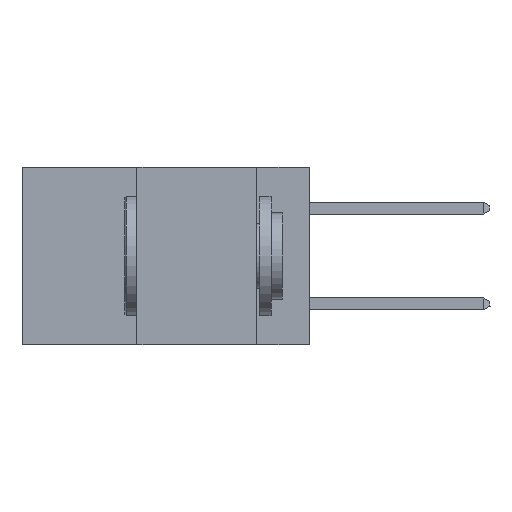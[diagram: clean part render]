
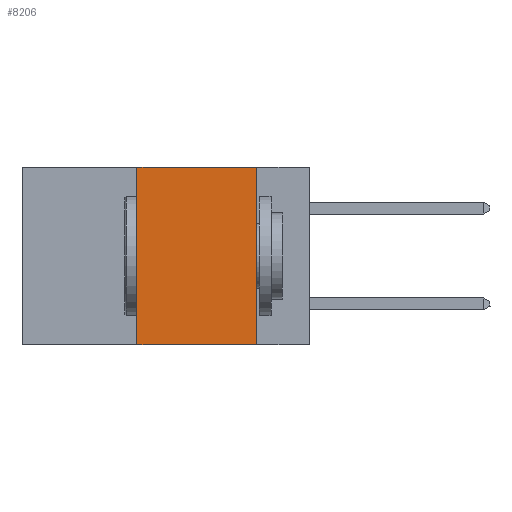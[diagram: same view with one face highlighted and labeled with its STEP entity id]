
A CAD part, left-side view. The second image highlights one B-rep face of the part: STEP entity #8206.
In plain terms, the highlighted planar face has unit normal (-1, 0, 0).
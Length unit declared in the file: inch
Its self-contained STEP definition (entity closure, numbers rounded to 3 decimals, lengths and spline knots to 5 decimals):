
#815 = VECTOR ( 'NONE', #8170, 39.37008 ) ;
#894 = VECTOR ( 'NONE', #13691, 39.37008 ) ;
#2569 = VECTOR ( 'NONE', #21278, 39.37008 ) ;
#2693 = CARTESIAN_POINT ( 'NONE',  ( 0., 0.6, -0.37 ) ) ;
#2923 = EDGE_CURVE ( 'NONE', #23876, #13328, #21551, .T. ) ;
#3193 = LINE ( 'NONE', #19257, #2569 ) ;
#3829 = CARTESIAN_POINT ( 'NONE',  ( 0., 0.6, 0. ) ) ;
#5627 = DIRECTION ( 'NONE',  ( 1., 0., 0. ) ) ;
#5824 = EDGE_CURVE ( 'NONE', #13328, #7468, #11287, .T. ) ;
#6142 = EDGE_CURVE ( 'NONE', #23876, #15051, #16605, .T. ) ;
#7190 = CARTESIAN_POINT ( 'NONE',  ( 0., 0.11, 0. ) ) ;
#7249 = ORIENTED_EDGE ( 'NONE', *, *, #15564, .F. ) ;
#7383 = CARTESIAN_POINT ( 'NONE',  ( 0., 0.36, 0. ) ) ;
#7468 = VERTEX_POINT ( 'NONE', #7190 ) ;
#8170 = DIRECTION ( 'NONE',  ( 0., 0., 1. ) ) ;
#8206 = ADVANCED_FACE ( 'NONE', ( #18088 ), #23444, .F. ) ;
#9370 = CARTESIAN_POINT ( 'NONE',  ( 0., 0.6, 0. ) ) ;
#10376 = CARTESIAN_POINT ( 'NONE',  ( 0., 0.36, 0. ) ) ;
#10899 = ORIENTED_EDGE ( 'NONE', *, *, #5824, .F. ) ;
#11287 = LINE ( 'NONE', #3829, #894 ) ;
#12989 = AXIS2_PLACEMENT_3D ( 'NONE', #9370, #5627, #19761 ) ;
#13328 = VERTEX_POINT ( 'NONE', #7383 ) ;
#13691 = DIRECTION ( 'NONE',  ( 0., -1., 0. ) ) ;
#14237 = CARTESIAN_POINT ( 'NONE',  ( 0., 0.36, -0.37 ) ) ;
#15051 = VERTEX_POINT ( 'NONE', #25964 ) ;
#15564 = EDGE_CURVE ( 'NONE', #7468, #15051, #3193, .T. ) ;
#16605 = LINE ( 'NONE', #2693, #18790 ) ;
#16943 = ORIENTED_EDGE ( 'NONE', *, *, #2923, .F. ) ;
#18088 = FACE_OUTER_BOUND ( 'NONE', #22813, .T. ) ;
#18790 = VECTOR ( 'NONE', #20882, 39.37008 ) ;
#19257 = CARTESIAN_POINT ( 'NONE',  ( 0., 0.11, 0. ) ) ;
#19761 = DIRECTION ( 'NONE',  ( 0., 0., -1. ) ) ;
#20882 = DIRECTION ( 'NONE',  ( 0., -1., 0. ) ) ;
#21278 = DIRECTION ( 'NONE',  ( 0., 0., -1. ) ) ;
#21551 = LINE ( 'NONE', #10376, #815 ) ;
#22066 = ORIENTED_EDGE ( 'NONE', *, *, #6142, .T. ) ;
#22813 = EDGE_LOOP ( 'NONE', ( #7249, #10899, #16943, #22066 ) ) ;
#23444 = PLANE ( 'NONE',  #12989 ) ;
#23876 = VERTEX_POINT ( 'NONE', #14237 ) ;
#25964 = CARTESIAN_POINT ( 'NONE',  ( 0., 0.11, -0.37 ) ) ;
